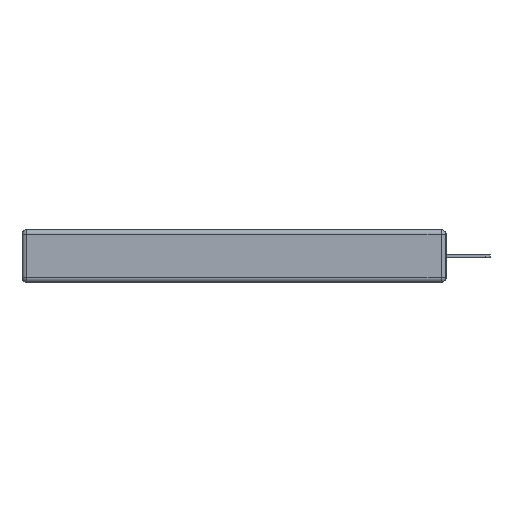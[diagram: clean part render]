
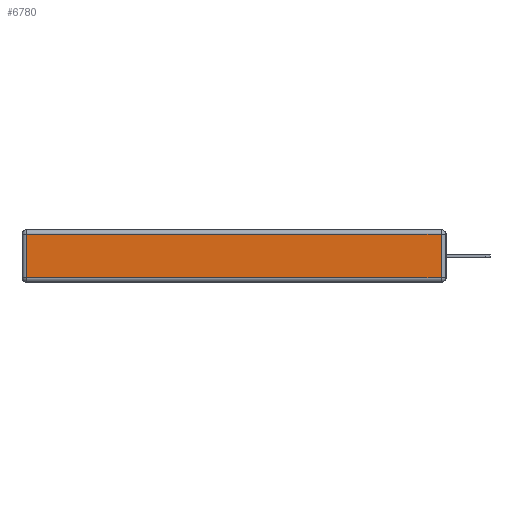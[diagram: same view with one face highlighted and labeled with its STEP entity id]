
A CAD part, left-side view. The second image highlights one B-rep face of the part: STEP entity #6780.
In plain terms, the highlighted planar face has unit normal (-1, 0, 0).
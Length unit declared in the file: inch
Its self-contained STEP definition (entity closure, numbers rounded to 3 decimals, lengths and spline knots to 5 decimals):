
#52 = CARTESIAN_POINT ( 'NONE',  ( 0., 0.03, -0.343 ) ) ;
#56 = VERTEX_POINT ( 'NONE', #11273 ) ;
#301 = EDGE_CURVE ( 'NONE', #11721, #15827, #14100, .T. ) ;
#2369 = ORIENTED_EDGE ( 'NONE', *, *, #15305, .T. ) ;
#3434 = DIRECTION ( 'NONE',  ( 0., 0., 1. ) ) ;
#4603 = CARTESIAN_POINT ( 'NONE',  ( 0., 0.03, -0.03 ) ) ;
#4703 = DIRECTION ( 'NONE',  ( 0., -1., 0. ) ) ;
#5777 = CARTESIAN_POINT ( 'NONE',  ( 0., 0., -0.343 ) ) ;
#6780 = ADVANCED_FACE ( 'NONE', ( #7385 ), #12847, .T. ) ;
#7385 = FACE_OUTER_BOUND ( 'NONE', #12385, .T. ) ;
#7500 = VECTOR ( 'NONE', #18947, 39.37008 ) ;
#9354 = ORIENTED_EDGE ( 'NONE', *, *, #24254, .T. ) ;
#10227 = EDGE_CURVE ( 'NONE', #23190, #56, #11766, .T. ) ;
#10271 = DIRECTION ( 'NONE',  ( 0., 1., 0. ) ) ;
#10577 = ORIENTED_EDGE ( 'NONE', *, *, #301, .T. ) ;
#11273 = CARTESIAN_POINT ( 'NONE',  ( 0., 2.72, -0.03 ) ) ;
#11721 = VERTEX_POINT ( 'NONE', #23276 ) ;
#11766 = LINE ( 'NONE', #12132, #22059 ) ;
#12132 = CARTESIAN_POINT ( 'NONE',  ( 0., 2.75, -0.03 ) ) ;
#12385 = EDGE_LOOP ( 'NONE', ( #10577, #9354, #15488, #2369 ) ) ;
#12847 = PLANE ( 'NONE',  #15273 ) ;
#12961 = DIRECTION ( 'NONE',  ( -1., 0., 0. ) ) ;
#14100 = LINE ( 'NONE', #21632, #21170 ) ;
#15152 = DIRECTION ( 'NONE',  ( 0., 0., -1. ) ) ;
#15273 = AXIS2_PLACEMENT_3D ( 'NONE', #5777, #12961, #3434 ) ;
#15305 = EDGE_CURVE ( 'NONE', #56, #11721, #17237, .T. ) ;
#15488 = ORIENTED_EDGE ( 'NONE', *, *, #10227, .T. ) ;
#15827 = VERTEX_POINT ( 'NONE', #23615 ) ;
#17237 = LINE ( 'NONE', #20689, #17282 ) ;
#17282 = VECTOR ( 'NONE', #15152, 39.37008 ) ;
#18947 = DIRECTION ( 'NONE',  ( 0., 0., 1. ) ) ;
#20689 = CARTESIAN_POINT ( 'NONE',  ( 0., 2.72, -0.343 ) ) ;
#21170 = VECTOR ( 'NONE', #4703, 39.37008 ) ;
#21632 = CARTESIAN_POINT ( 'NONE',  ( 0., 0., -0.313 ) ) ;
#22059 = VECTOR ( 'NONE', #10271, 39.37008 ) ;
#23190 = VERTEX_POINT ( 'NONE', #4603 ) ;
#23276 = CARTESIAN_POINT ( 'NONE',  ( 0., 2.72, -0.313 ) ) ;
#23615 = CARTESIAN_POINT ( 'NONE',  ( 0., 0.03, -0.313 ) ) ;
#24158 = LINE ( 'NONE', #52, #7500 ) ;
#24254 = EDGE_CURVE ( 'NONE', #15827, #23190, #24158, .T. ) ;
